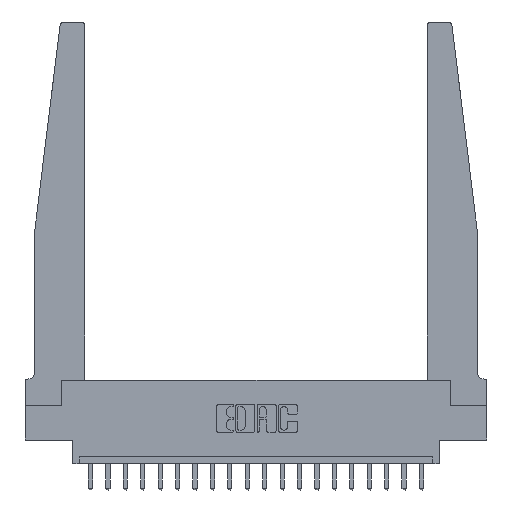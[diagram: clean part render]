
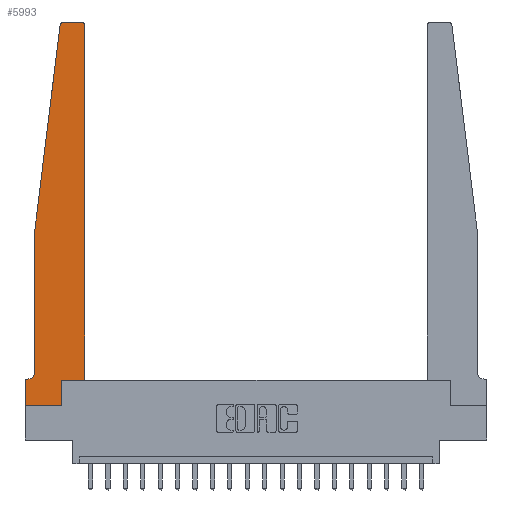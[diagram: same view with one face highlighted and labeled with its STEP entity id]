
A CAD part, top view. The second image highlights one B-rep face of the part: STEP entity #5993.
In plain terms, the highlighted planar face has unit normal (0, 0, 1).
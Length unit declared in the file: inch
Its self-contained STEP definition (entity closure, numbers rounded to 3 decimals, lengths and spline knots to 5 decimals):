
#382 = VECTOR ( 'NONE', #754, 39.37008 ) ;
#636 = CARTESIAN_POINT ( 'NONE',  ( 0.065, 0.2375, 0.37 ) ) ;
#754 = DIRECTION ( 'NONE',  ( 0., 1., 0. ) ) ;
#1776 = EDGE_CURVE ( 'NONE', #5791, #15693, #15153, .T. ) ;
#1790 = CIRCLE ( 'NONE', #13563, 0.05 ) ;
#2012 = CARTESIAN_POINT ( 'NONE',  ( 0.425, 0.18, 0.37 ) ) ;
#2165 = DIRECTION ( 'NONE',  ( -1., 0., 0. ) ) ;
#2485 = VECTOR ( 'NONE', #20411, 39.37008 ) ;
#2615 = CARTESIAN_POINT ( 'NONE',  ( 0.2605, 0.18, 0.37 ) ) ;
#2621 = FACE_OUTER_BOUND ( 'NONE', #8861, .T. ) ;
#2750 = VECTOR ( 'NONE', #7274, 39.37008 ) ;
#2752 = LINE ( 'NONE', #13805, #14430 ) ;
#2933 = VERTEX_POINT ( 'NONE', #8366 ) ;
#3038 = VERTEX_POINT ( 'NONE', #3735 ) ;
#3436 = EDGE_CURVE ( 'NONE', #17756, #3038, #20795, .T. ) ;
#3735 = CARTESIAN_POINT ( 'NONE',  ( 0.24675, 2.72367, 0.37 ) ) ;
#3879 = ORIENTED_EDGE ( 'NONE', *, *, #1776, .T. ) ;
#4222 = DIRECTION ( 'NONE',  ( 0., 0., 1. ) ) ;
#4299 = LINE ( 'NONE', #15531, #2485 ) ;
#4844 = EDGE_CURVE ( 'NONE', #18091, #5791, #2752, .T. ) ;
#5697 = LINE ( 'NONE', #5799, #7044 ) ;
#5735 = ORIENTED_EDGE ( 'NONE', *, *, #11537, .T. ) ;
#5791 = VERTEX_POINT ( 'NONE', #18456 ) ;
#5799 = CARTESIAN_POINT ( 'NONE',  ( 0., 0., 0.37 ) ) ;
#5993 = ADVANCED_FACE ( 'NONE', ( #2621 ), #12101, .T. ) ;
#6005 = VERTEX_POINT ( 'NONE', #636 ) ;
#6422 = CARTESIAN_POINT ( 'NONE',  ( 0., 0.1875, 0.37 ) ) ;
#6427 = DIRECTION ( 'NONE',  ( 0., -1., 0. ) ) ;
#6627 = ORIENTED_EDGE ( 'NONE', *, *, #4844, .T. ) ;
#6639 = LINE ( 'NONE', #14496, #11903 ) ;
#7044 = VECTOR ( 'NONE', #15554, 39.37008 ) ;
#7071 = DIRECTION ( 'NONE',  ( 0., 0., 1. ) ) ;
#7274 = DIRECTION ( 'NONE',  ( 0., 1., 0. ) ) ;
#7497 = VERTEX_POINT ( 'NONE', #14854 ) ;
#7501 = LINE ( 'NONE', #9173, #13869 ) ;
#7702 = DIRECTION ( 'NONE',  ( 1., 0., 0. ) ) ;
#7874 = VECTOR ( 'NONE', #19141, 39.37008 ) ;
#8022 = VECTOR ( 'NONE', #18208, 39.37008 ) ;
#8168 = VERTEX_POINT ( 'NONE', #6422 ) ;
#8272 = DIRECTION ( 'NONE',  ( 1., 0., 0. ) ) ;
#8366 = CARTESIAN_POINT ( 'NONE',  ( 0.015, 0.1875, 0.37 ) ) ;
#8719 = LINE ( 'NONE', #2615, #2750 ) ;
#8759 = AXIS2_PLACEMENT_3D ( 'NONE', #12204, #7071, #19785 ) ;
#8797 = EDGE_CURVE ( 'NONE', #15693, #19803, #15870, .T. ) ;
#8861 = EDGE_LOOP ( 'NONE', ( #10364, #12343, #5735, #18040, #12594, #17145, #12779, #19818, #14790, #6627, #3879, #15613 ) ) ;
#9089 = CARTESIAN_POINT ( 'NONE',  ( 0.395, 2.75, 0.37 ) ) ;
#9173 = CARTESIAN_POINT ( 'NONE',  ( 0.065, 0.1875, 0.37 ) ) ;
#9403 = EDGE_CURVE ( 'NONE', #7497, #6005, #6639, .T. ) ;
#9758 = EDGE_CURVE ( 'NONE', #19803, #17756, #4299, .T. ) ;
#9995 = VERTEX_POINT ( 'NONE', #16782 ) ;
#10364 = ORIENTED_EDGE ( 'NONE', *, *, #9758, .T. ) ;
#10403 = CARTESIAN_POINT ( 'NONE',  ( 0.2605, 0.18, 0.37 ) ) ;
#10746 = EDGE_CURVE ( 'NONE', #6005, #2933, #1790, .T. ) ;
#11537 = EDGE_CURVE ( 'NONE', #3038, #7497, #17867, .T. ) ;
#11541 = DIRECTION ( 'NONE',  ( 0., 0., 1. ) ) ;
#11719 = AXIS2_PLACEMENT_3D ( 'NONE', #18635, #4222, #19898 ) ;
#11903 = VECTOR ( 'NONE', #6427, 39.37008 ) ;
#12100 = VERTEX_POINT ( 'NONE', #16023 ) ;
#12101 = PLANE ( 'NONE',  #8759 ) ;
#12204 = CARTESIAN_POINT ( 'NONE',  ( 0., 0.1875, 0.37 ) ) ;
#12343 = ORIENTED_EDGE ( 'NONE', *, *, #3436, .T. ) ;
#12534 = DIRECTION ( 'NONE',  ( -1., 0., 0. ) ) ;
#12594 = ORIENTED_EDGE ( 'NONE', *, *, #10746, .T. ) ;
#12722 = CARTESIAN_POINT ( 'NONE',  ( 0.065, 1.25, 0.37 ) ) ;
#12779 = ORIENTED_EDGE ( 'NONE', *, *, #15884, .T. ) ;
#12918 = CARTESIAN_POINT ( 'NONE',  ( 0.27653, 2.75, 0.37 ) ) ;
#13563 = AXIS2_PLACEMENT_3D ( 'NONE', #16571, #19740, #2165 ) ;
#13805 = CARTESIAN_POINT ( 'NONE',  ( 0.425, 0.18, 0.37 ) ) ;
#13869 = VECTOR ( 'NONE', #12534, 39.37008 ) ;
#14430 = VECTOR ( 'NONE', #7702, 39.37008 ) ;
#14496 = CARTESIAN_POINT ( 'NONE',  ( 0.065, 1.25, 0.37 ) ) ;
#14790 = ORIENTED_EDGE ( 'NONE', *, *, #18904, .T. ) ;
#14854 = CARTESIAN_POINT ( 'NONE',  ( 0.065, 1.25, 0.37 ) ) ;
#15048 = LINE ( 'NONE', #16406, #8022 ) ;
#15153 = LINE ( 'NONE', #2012, #382 ) ;
#15531 = CARTESIAN_POINT ( 'NONE',  ( 0.25, 2.75, 0.37 ) ) ;
#15554 = DIRECTION ( 'NONE',  ( 1., 0., 0. ) ) ;
#15613 = ORIENTED_EDGE ( 'NONE', *, *, #8797, .T. ) ;
#15693 = VERTEX_POINT ( 'NONE', #17471 ) ;
#15870 = CIRCLE ( 'NONE', #18915, 0.03 ) ;
#15884 = EDGE_CURVE ( 'NONE', #8168, #12100, #15048, .T. ) ;
#15947 = EDGE_CURVE ( 'NONE', #12100, #9995, #5697, .T. ) ;
#16023 = CARTESIAN_POINT ( 'NONE',  ( 0., 0., 0.37 ) ) ;
#16406 = CARTESIAN_POINT ( 'NONE',  ( 0., 0., 0.37 ) ) ;
#16571 = CARTESIAN_POINT ( 'NONE',  ( 0.015, 0.2375, 0.37 ) ) ;
#16676 = CARTESIAN_POINT ( 'NONE',  ( 0.395, 2.72, 0.37 ) ) ;
#16782 = CARTESIAN_POINT ( 'NONE',  ( 0.2605, 0., 0.37 ) ) ;
#17145 = ORIENTED_EDGE ( 'NONE', *, *, #20188, .T. ) ;
#17471 = CARTESIAN_POINT ( 'NONE',  ( 0.425, 2.72, 0.37 ) ) ;
#17756 = VERTEX_POINT ( 'NONE', #12918 ) ;
#17867 = LINE ( 'NONE', #12722, #7874 ) ;
#18040 = ORIENTED_EDGE ( 'NONE', *, *, #9403, .T. ) ;
#18091 = VERTEX_POINT ( 'NONE', #10403 ) ;
#18208 = DIRECTION ( 'NONE',  ( 0., -1., 0. ) ) ;
#18456 = CARTESIAN_POINT ( 'NONE',  ( 0.425, 0.18, 0.37 ) ) ;
#18635 = CARTESIAN_POINT ( 'NONE',  ( 0.27653, 2.72, 0.37 ) ) ;
#18904 = EDGE_CURVE ( 'NONE', #9995, #18091, #8719, .T. ) ;
#18915 = AXIS2_PLACEMENT_3D ( 'NONE', #16676, #11541, #8272 ) ;
#19141 = DIRECTION ( 'NONE',  ( -0.122, -0.992, 0. ) ) ;
#19740 = DIRECTION ( 'NONE',  ( 0., 0., -1. ) ) ;
#19785 = DIRECTION ( 'NONE',  ( 1., 0., 0. ) ) ;
#19803 = VERTEX_POINT ( 'NONE', #9089 ) ;
#19818 = ORIENTED_EDGE ( 'NONE', *, *, #15947, .T. ) ;
#19898 = DIRECTION ( 'NONE',  ( 1., 0., 0. ) ) ;
#20188 = EDGE_CURVE ( 'NONE', #2933, #8168, #7501, .T. ) ;
#20411 = DIRECTION ( 'NONE',  ( -1., 0., 0. ) ) ;
#20795 = CIRCLE ( 'NONE', #11719, 0.03 ) ;
